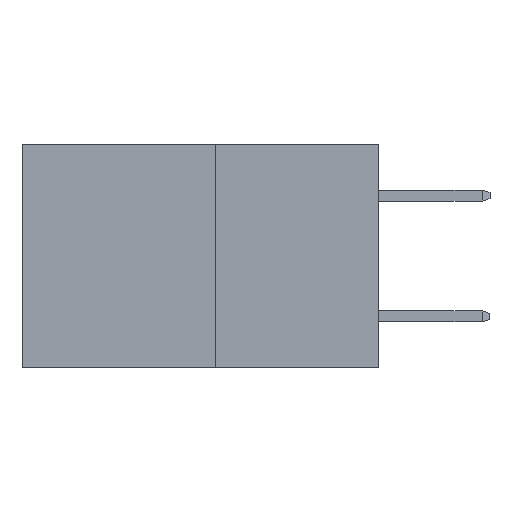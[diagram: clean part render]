
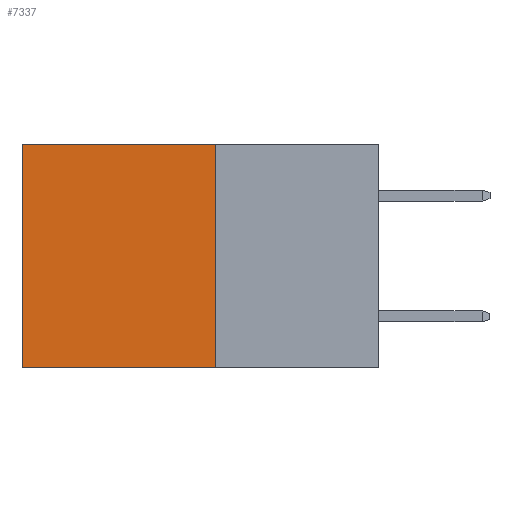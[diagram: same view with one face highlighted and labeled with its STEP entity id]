
A CAD part, left-side view. The second image highlights one B-rep face of the part: STEP entity #7337.
In plain terms, the highlighted planar face has unit normal (-1, 0, 0).
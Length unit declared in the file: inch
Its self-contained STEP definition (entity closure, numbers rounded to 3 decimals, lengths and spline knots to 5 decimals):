
#224 = EDGE_CURVE ( 'NONE', #1951, #6160, #4390, .T. ) ;
#621 = LINE ( 'NONE', #3383, #4275 ) ;
#1852 = CARTESIAN_POINT ( 'NONE',  ( 0.277, 0.27, -0.37 ) ) ;
#1893 = FACE_OUTER_BOUND ( 'NONE', #8970, .T. ) ;
#1903 = VECTOR ( 'NONE', #1984, 39.37008 ) ;
#1951 = VERTEX_POINT ( 'NONE', #3823 ) ;
#1984 = DIRECTION ( 'NONE',  ( 0., 1., 0. ) ) ;
#2319 = VECTOR ( 'NONE', #3508, 39.37008 ) ;
#2497 = VECTOR ( 'NONE', #3164, 39.37008 ) ;
#2668 = AXIS2_PLACEMENT_3D ( 'NONE', #2977, #8418, #4441 ) ;
#2977 = CARTESIAN_POINT ( 'NONE',  ( 0.277, 0.27, -0.37 ) ) ;
#3164 = DIRECTION ( 'NONE',  ( 0., 0., -1. ) ) ;
#3172 = DIRECTION ( 'NONE',  ( 0., 0., -1. ) ) ;
#3188 = EDGE_CURVE ( 'NONE', #7004, #3529, #621, .T. ) ;
#3383 = CARTESIAN_POINT ( 'NONE',  ( 0.277, 0.59, -0.37 ) ) ;
#3508 = DIRECTION ( 'NONE',  ( 0., 1., 0. ) ) ;
#3529 = VERTEX_POINT ( 'NONE', #5957 ) ;
#3823 = CARTESIAN_POINT ( 'NONE',  ( 0.277, 0.27, 0. ) ) ;
#3977 = CARTESIAN_POINT ( 'NONE',  ( 0.277, 0.27, -0.37 ) ) ;
#4216 = LINE ( 'NONE', #8215, #2319 ) ;
#4275 = VECTOR ( 'NONE', #3172, 39.37008 ) ;
#4390 = LINE ( 'NONE', #1852, #2497 ) ;
#4441 = DIRECTION ( 'NONE',  ( 0., 0., -1. ) ) ;
#5062 = EDGE_CURVE ( 'NONE', #1951, #7004, #5627, .T. ) ;
#5473 = ORIENTED_EDGE ( 'NONE', *, *, #3188, .T. ) ;
#5627 = LINE ( 'NONE', #6814, #1903 ) ;
#5709 = ORIENTED_EDGE ( 'NONE', *, *, #6331, .F. ) ;
#5957 = CARTESIAN_POINT ( 'NONE',  ( 0.277, 0.59, -0.37 ) ) ;
#6160 = VERTEX_POINT ( 'NONE', #3977 ) ;
#6331 = EDGE_CURVE ( 'NONE', #6160, #3529, #4216, .T. ) ;
#6735 = ORIENTED_EDGE ( 'NONE', *, *, #224, .F. ) ;
#6814 = CARTESIAN_POINT ( 'NONE',  ( 0.277, 0.27, 0. ) ) ;
#7004 = VERTEX_POINT ( 'NONE', #8698 ) ;
#7255 = ORIENTED_EDGE ( 'NONE', *, *, #5062, .T. ) ;
#7337 = ADVANCED_FACE ( 'NONE', ( #1893 ), #7773, .F. ) ;
#7773 = PLANE ( 'NONE',  #2668 ) ;
#8215 = CARTESIAN_POINT ( 'NONE',  ( 0.277, 0.27, -0.37 ) ) ;
#8418 = DIRECTION ( 'NONE',  ( 1., 0., 0. ) ) ;
#8698 = CARTESIAN_POINT ( 'NONE',  ( 0.277, 0.59, 0. ) ) ;
#8970 = EDGE_LOOP ( 'NONE', ( #5473, #5709, #6735, #7255 ) ) ;
